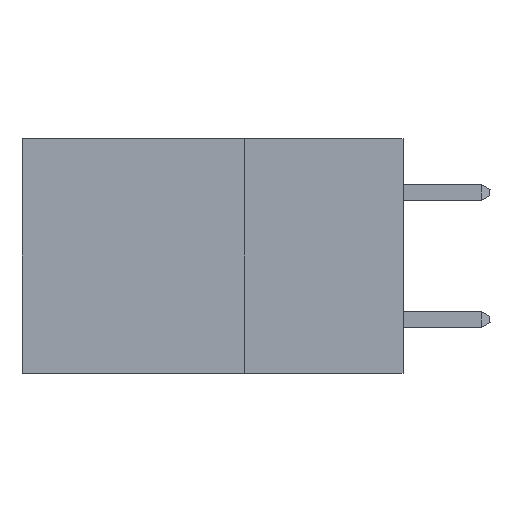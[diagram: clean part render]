
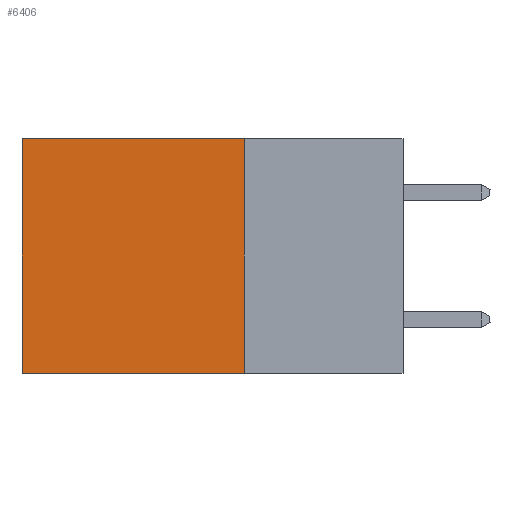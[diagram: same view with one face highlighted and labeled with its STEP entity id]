
A CAD part, left-side view. The second image highlights one B-rep face of the part: STEP entity #6406.
In plain terms, the highlighted planar face has unit normal (-1, 0, 0).
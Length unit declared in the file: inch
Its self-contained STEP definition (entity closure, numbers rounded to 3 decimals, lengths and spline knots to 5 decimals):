
#202 = ORIENTED_EDGE ( 'NONE', *, *, #8354, .T. ) ;
#692 = EDGE_CURVE ( 'NONE', #1966, #10710, #6696, .T. ) ;
#846 = ORIENTED_EDGE ( 'NONE', *, *, #11280, .F. ) ;
#1006 = AXIS2_PLACEMENT_3D ( 'NONE', #7670, #8564, #3246 ) ;
#1103 = VERTEX_POINT ( 'NONE', #1620 ) ;
#1202 = EDGE_LOOP ( 'NONE', ( #1366, #846, #2508, #202 ) ) ;
#1349 = EDGE_CURVE ( 'NONE', #8979, #1103, #6816, .T. ) ;
#1366 = ORIENTED_EDGE ( 'NONE', *, *, #692, .T. ) ;
#1443 = PLANE ( 'NONE',  #1006 ) ;
#1448 = VECTOR ( 'NONE', #6858, 39.37008 ) ;
#1620 = CARTESIAN_POINT ( 'NONE',  ( 0.2875, 0.25, -0.37 ) ) ;
#1948 = VECTOR ( 'NONE', #9895, 39.37008 ) ;
#1966 = VERTEX_POINT ( 'NONE', #10930 ) ;
#2508 = ORIENTED_EDGE ( 'NONE', *, *, #1349, .F. ) ;
#3246 = DIRECTION ( 'NONE',  ( 0., 0., -1. ) ) ;
#3813 = LINE ( 'NONE', #9509, #1448 ) ;
#4663 = DIRECTION ( 'NONE',  ( 0., 0., -1. ) ) ;
#5163 = CARTESIAN_POINT ( 'NONE',  ( 0.2875, 0.6, -0.37 ) ) ;
#5554 = CARTESIAN_POINT ( 'NONE',  ( 0.2875, 0.25, 0. ) ) ;
#6406 = ADVANCED_FACE ( 'NONE', ( #8465 ), #1443, .F. ) ;
#6696 = LINE ( 'NONE', #9022, #1948 ) ;
#6816 = LINE ( 'NONE', #5554, #11205 ) ;
#6858 = DIRECTION ( 'NONE',  ( 0., 1., 0. ) ) ;
#7016 = LINE ( 'NONE', #10426, #8831 ) ;
#7670 = CARTESIAN_POINT ( 'NONE',  ( 0.2875, 0.25, 0. ) ) ;
#8354 = EDGE_CURVE ( 'NONE', #8979, #1966, #7016, .T. ) ;
#8465 = FACE_OUTER_BOUND ( 'NONE', #1202, .T. ) ;
#8564 = DIRECTION ( 'NONE',  ( 1., 0., 0. ) ) ;
#8725 = DIRECTION ( 'NONE',  ( 0., 1., 0. ) ) ;
#8831 = VECTOR ( 'NONE', #8725, 39.37008 ) ;
#8979 = VERTEX_POINT ( 'NONE', #11238 ) ;
#9022 = CARTESIAN_POINT ( 'NONE',  ( 0.2875, 0.6, 0. ) ) ;
#9509 = CARTESIAN_POINT ( 'NONE',  ( 0.2875, 0.25, -0.37 ) ) ;
#9895 = DIRECTION ( 'NONE',  ( 0., 0., -1. ) ) ;
#10426 = CARTESIAN_POINT ( 'NONE',  ( 0.2875, 0.25, 0. ) ) ;
#10710 = VERTEX_POINT ( 'NONE', #5163 ) ;
#10930 = CARTESIAN_POINT ( 'NONE',  ( 0.2875, 0.6, 0. ) ) ;
#11205 = VECTOR ( 'NONE', #4663, 39.37008 ) ;
#11238 = CARTESIAN_POINT ( 'NONE',  ( 0.2875, 0.25, 0. ) ) ;
#11280 = EDGE_CURVE ( 'NONE', #1103, #10710, #3813, .T. ) ;
